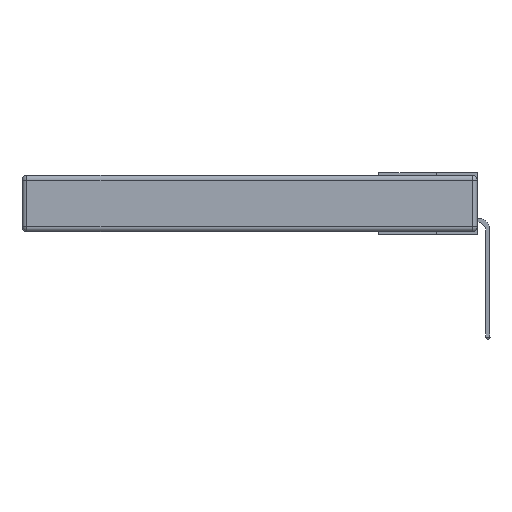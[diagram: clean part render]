
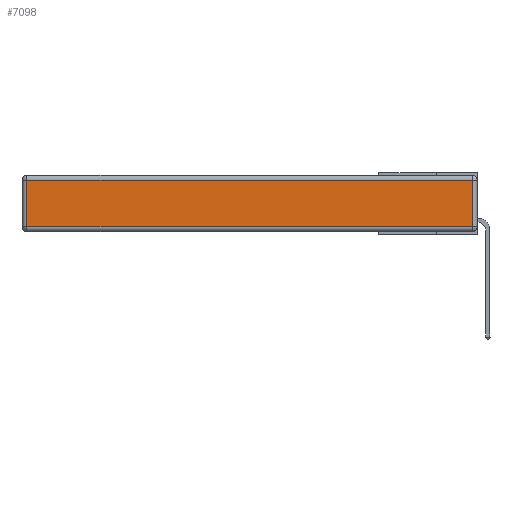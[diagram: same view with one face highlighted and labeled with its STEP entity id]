
A CAD part, left-side view. The second image highlights one B-rep face of the part: STEP entity #7098.
In plain terms, the highlighted planar face has unit normal (-1, 0, 0).
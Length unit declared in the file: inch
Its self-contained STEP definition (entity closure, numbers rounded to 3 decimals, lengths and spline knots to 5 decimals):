
#780 = EDGE_CURVE ( 'NONE', #9339, #13161, #23007, .T. ) ;
#912 = ORIENTED_EDGE ( 'NONE', *, *, #10665, .T. ) ;
#1705 = LINE ( 'NONE', #22869, #28146 ) ;
#4078 = CARTESIAN_POINT ( 'NONE',  ( 0., 0.03, -0.313 ) ) ;
#4093 = EDGE_CURVE ( 'NONE', #13161, #11306, #1705, .T. ) ;
#5387 = ORIENTED_EDGE ( 'NONE', *, *, #7231, .T. ) ;
#5683 = DIRECTION ( 'NONE',  ( 0., -1., 0. ) ) ;
#7098 = ADVANCED_FACE ( 'NONE', ( #10542 ), #17863, .T. ) ;
#7231 = EDGE_CURVE ( 'NONE', #7559, #9339, #8170, .T. ) ;
#7424 = DIRECTION ( 'NONE',  ( -1., 0., 0. ) ) ;
#7559 = VERTEX_POINT ( 'NONE', #24669 ) ;
#8170 = LINE ( 'NONE', #10886, #20223 ) ;
#9339 = VERTEX_POINT ( 'NONE', #11376 ) ;
#10542 = FACE_OUTER_BOUND ( 'NONE', #30933, .T. ) ;
#10665 = EDGE_CURVE ( 'NONE', #11306, #7559, #17512, .T. ) ;
#10886 = CARTESIAN_POINT ( 'NONE',  ( 0., 2.72, -0.343 ) ) ;
#11306 = VERTEX_POINT ( 'NONE', #29141 ) ;
#11376 = CARTESIAN_POINT ( 'NONE',  ( 0., 2.72, -0.313 ) ) ;
#12006 = ORIENTED_EDGE ( 'NONE', *, *, #4093, .T. ) ;
#13161 = VERTEX_POINT ( 'NONE', #4078 ) ;
#14630 = ORIENTED_EDGE ( 'NONE', *, *, #780, .T. ) ;
#14868 = VECTOR ( 'NONE', #5683, 39.37008 ) ;
#15869 = DIRECTION ( 'NONE',  ( 0., 0., 1. ) ) ;
#17512 = LINE ( 'NONE', #29742, #24861 ) ;
#17863 = PLANE ( 'NONE',  #25946 ) ;
#20223 = VECTOR ( 'NONE', #28156, 39.37008 ) ;
#20344 = CARTESIAN_POINT ( 'NONE',  ( 0., 0., -0.343 ) ) ;
#22869 = CARTESIAN_POINT ( 'NONE',  ( 0., 0.03, -0.343 ) ) ;
#23007 = LINE ( 'NONE', #30276, #14868 ) ;
#24669 = CARTESIAN_POINT ( 'NONE',  ( 0., 2.72, -0.03 ) ) ;
#24861 = VECTOR ( 'NONE', #29636, 39.37008 ) ;
#25946 = AXIS2_PLACEMENT_3D ( 'NONE', #20344, #7424, #15869 ) ;
#27867 = DIRECTION ( 'NONE',  ( 0., 0., 1. ) ) ;
#28146 = VECTOR ( 'NONE', #27867, 39.37008 ) ;
#28156 = DIRECTION ( 'NONE',  ( 0., 0., -1. ) ) ;
#29141 = CARTESIAN_POINT ( 'NONE',  ( 0., 0.03, -0.03 ) ) ;
#29636 = DIRECTION ( 'NONE',  ( 0., 1., 0. ) ) ;
#29742 = CARTESIAN_POINT ( 'NONE',  ( 0., 2.75, -0.03 ) ) ;
#30276 = CARTESIAN_POINT ( 'NONE',  ( 0., 0., -0.313 ) ) ;
#30933 = EDGE_LOOP ( 'NONE', ( #14630, #12006, #912, #5387 ) ) ;
